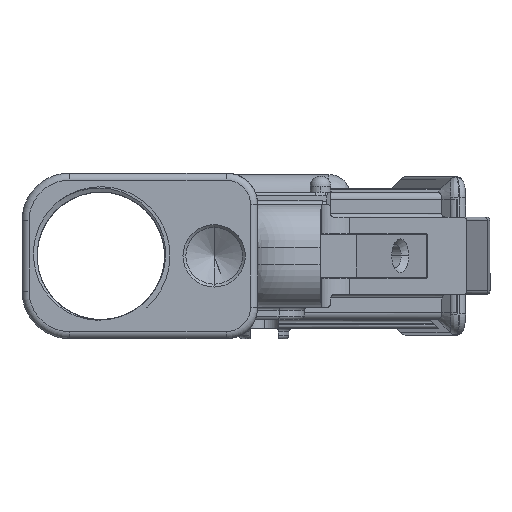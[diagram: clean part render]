
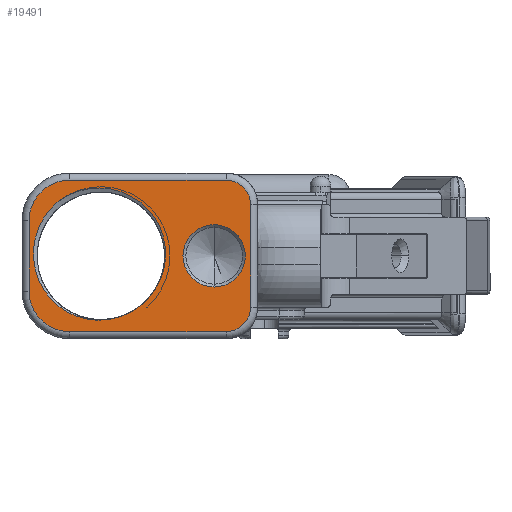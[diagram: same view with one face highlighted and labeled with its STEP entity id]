
A CAD part, left-side view. The second image highlights one B-rep face of the part: STEP entity #19491.
In plain terms, the highlighted planar face has unit normal (-1, 0, 0).
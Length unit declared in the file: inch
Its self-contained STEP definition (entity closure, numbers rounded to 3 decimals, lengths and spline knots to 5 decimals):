
#1840=DIRECTION('',(0.,0.,-1.));
#1841=VECTOR('',#1840,0.90625);
#1842=CARTESIAN_POINT('',(-7.565,-0.442,0.45313));
#1843=LINE('',#1842,#1841);
#1863=DIRECTION('',(0.,-1.,0.));
#1864=VECTOR('',#1863,1.38327);
#1865=CARTESIAN_POINT('',(-7.565,1.15661,0.66847));
#1866=LINE('',#1865,#1864);
#1882=DIRECTION('',(0.,0.,1.));
#1883=VECTOR('',#1882,0.62416);
#1884=CARTESIAN_POINT('',(-7.565,1.513,-0.31208));
#1885=LINE('',#1884,#1883);
#1890=CARTESIAN_POINT('',(-7.565,1.15661,-0.31208));
#1891=DIRECTION('',(-1.,0.,0.));
#1892=DIRECTION('',(0.,1.,0.));
#1893=AXIS2_PLACEMENT_3D('',#1890,#1891,#1892);
#1895=CARTESIAN_POINT('',(-7.565,1.15661,0.31208));
#1896=DIRECTION('',(-1.,0.,0.));
#1897=DIRECTION('',(0.,0.,1.));
#1898=AXIS2_PLACEMENT_3D('',#1895,#1896,#1897);
#1900=CARTESIAN_POINT('',(-7.565,-0.22666,0.45313));
#1901=DIRECTION('',(-1.,0.,0.));
#1902=DIRECTION('',(0.,-1.,0.));
#1903=AXIS2_PLACEMENT_3D('',#1900,#1901,#1902);
#1905=CARTESIAN_POINT('',(-7.565,-0.22666,-0.45313));
#1906=DIRECTION('',(-1.,0.,0.));
#1907=DIRECTION('',(0.,0.,-1.));
#1908=AXIS2_PLACEMENT_3D('',#1905,#1906,#1907);
#1910=CARTESIAN_POINT('',(-7.565,-0.1205,0.));
#1911=DIRECTION('',(1.,0.,0.));
#1912=DIRECTION('',(0.,0.,-1.));
#1913=AXIS2_PLACEMENT_3D('',#1910,#1911,#1912);
#1915=CARTESIAN_POINT('',(-7.565,-0.1205,0.));
#1916=DIRECTION('',(1.,0.,0.));
#1917=DIRECTION('',(0.,0.,1.));
#1918=AXIS2_PLACEMENT_3D('',#1915,#1916,#1917);
#1920=CARTESIAN_POINT('',(-7.565,0.8795,0.));
#1921=DIRECTION('',(1.,0.,0.));
#1922=DIRECTION('',(0.,-0.864,-0.503));
#1923=AXIS2_PLACEMENT_3D('',#1920,#1921,#1922);
#1925=DIRECTION('',(0.,1.,0.));
#1926=VECTOR('',#1925,1.38327);
#1927=CARTESIAN_POINT('',(-7.565,-0.22666,-0.66847));
#1928=LINE('',#1927,#1926);
#9167=CARTESIAN_POINT('',(-7.565,0.39331,-0.28289));
#9168=CARTESIAN_POINT('',(-7.565,0.37309,-0.2505));
#9169=CARTESIAN_POINT('',(-7.565,0.33995,-0.18304));
#9170=CARTESIAN_POINT('',(-7.565,0.31075,-0.07319));
#9171=CARTESIAN_POINT('',(-7.565,0.3044,0.04239));
#9172=CARTESIAN_POINT('',(-7.565,0.32039,0.15424));
#9173=CARTESIAN_POINT('',(-7.565,0.35858,0.26326));
#9174=CARTESIAN_POINT('',(-7.565,0.41751,0.36218));
#9175=CARTESIAN_POINT('',(-7.565,0.49489,0.44785));
#9176=CARTESIAN_POINT('',(-7.565,0.58856,0.51755));
#9177=CARTESIAN_POINT('',(-7.565,0.69295,0.56736));
#9178=CARTESIAN_POINT('',(-7.565,0.80785,0.5965));
#9179=CARTESIAN_POINT('',(-7.565,0.92518,0.60224));
#9180=CARTESIAN_POINT('',(-7.565,1.04407,0.58485));
#9181=CARTESIAN_POINT('',(-7.565,1.15676,0.54436));
#9182=CARTESIAN_POINT('',(-7.565,1.22454,0.50384));
#9183=CARTESIAN_POINT('',(-7.565,1.25678,0.47993));
#9207=CARTESIAN_POINT('',(-7.565,1.25678,0.47993));
#9208=CARTESIAN_POINT('',(-7.565,1.28795,0.45398));
#9209=CARTESIAN_POINT('',(-7.565,1.34373,0.39735));
#9210=CARTESIAN_POINT('',(-7.565,1.40926,
0.29779));
#9211=CARTESIAN_POINT('',(-7.565,1.45394,
0.18707));
#9212=CARTESIAN_POINT('',(-7.565,1.47587,
0.07176));
#9213=CARTESIAN_POINT('',(-7.565,1.4752,
-0.04651));
#9214=CARTESIAN_POINT('',(-7.565,1.4511,
-0.16151));
#9215=CARTESIAN_POINT('',(-7.565,1.4054,
-0.26861));
#9216=CARTESIAN_POINT('',(-7.565,1.339,
-0.36526));
#9217=CARTESIAN_POINT('',(-7.565,1.25645,
-0.44572));
#9218=CARTESIAN_POINT('',(-7.565,1.15841,
-0.50888));
#9219=CARTESIAN_POINT('',(-7.565,1.05132,
-0.55049));
#9220=CARTESIAN_POINT('',(-7.565,0.93705,
-0.5704));
#9221=CARTESIAN_POINT('',(-7.565,0.82106,
-0.56679));
#9222=CARTESIAN_POINT('',(-7.565,0.7483,
-0.5495));
#9223=CARTESIAN_POINT('',(-7.565,0.71257,
-0.53715));
#9616=CARTESIAN_POINT('',(-7.565,1.25678,0.47993));
#15622=CARTESIAN_POINT('',(-7.565,0.39331,-0.28289));
#15623=CARTESIAN_POINT('',(-7.565,0.71256,-0.53716));
#15624=VERTEX_POINT('',#15622);
#15625=VERTEX_POINT('',#15623);
#16979=VERTEX_POINT('',#9616);
#17004=CARTESIAN_POINT('',(-7.565,-0.22666,-0.66847));
#17005=CARTESIAN_POINT('',(-7.565,1.15661,-0.66847));
#17006=VERTEX_POINT('',#17004);
#17007=VERTEX_POINT('',#17005);
#17008=CARTESIAN_POINT('',(-7.565,-0.442,-0.45313));
#17009=VERTEX_POINT('',#17008);
#17010=CARTESIAN_POINT('',(-7.565,-0.442,0.45313));
#17011=VERTEX_POINT('',#17010);
#17012=CARTESIAN_POINT('',(-7.565,-0.22666,0.66847));
#17013=VERTEX_POINT('',#17012);
#17014=CARTESIAN_POINT('',(-7.565,1.15661,0.66847));
#17015=VERTEX_POINT('',#17014);
#17016=CARTESIAN_POINT('',(-7.565,1.513,0.31208));
#17017=VERTEX_POINT('',#17016);
#17018=CARTESIAN_POINT('',(-7.565,1.513,-0.31208));
#17019=VERTEX_POINT('',#17018);
#17020=CARTESIAN_POINT('',(-7.565,-0.1205,-0.275));
#17021=CARTESIAN_POINT('',(-7.565,-0.1205,0.275));
#17022=VERTEX_POINT('',#17020);
#17023=VERTEX_POINT('',#17021);
#19459=CARTESIAN_POINT('',(-7.565,0.,-0.45313));
#19460=DIRECTION('',(-1.,0.,0.));
#19461=DIRECTION('',(0.,0.,1.));
#19462=AXIS2_PLACEMENT_3D('',#19459,#19460,#19461);
#19463=PLANE('',#19462);
#19465=ORIENTED_EDGE('',*,*,#19464,.T.);
#19467=ORIENTED_EDGE('',*,*,#19466,.F.);
#19468=ORIENTED_EDGE('',*,*,#19450,.T.);
#19469=ORIENTED_EDGE('',*,*,#19439,.F.);
#19470=ORIENTED_EDGE('',*,*,#19424,.T.);
#19471=ORIENTED_EDGE('',*,*,#19409,.F.);
#19472=ORIENTED_EDGE('',*,*,#19394,.T.);
#19474=ORIENTED_EDGE('',*,*,#19473,.F.);
#19475=EDGE_LOOP('',(#19465,#19467,#19468,#19469,#19470,#19471,#19472,#19474));
#19476=FACE_OUTER_BOUND('',#19475,.F.);
#19478=ORIENTED_EDGE('',*,*,#19477,.F.);
#19480=ORIENTED_EDGE('',*,*,#19479,.F.);
#19481=EDGE_LOOP('',(#19478,#19480));
#19482=FACE_BOUND('',#19481,.F.);
#19484=ORIENTED_EDGE('',*,*,#19483,.T.);
#19486=ORIENTED_EDGE('',*,*,#19485,.F.);
#19488=ORIENTED_EDGE('',*,*,#19487,.T.);
#19489=EDGE_LOOP('',(#19484,#19486,#19488));
#19490=FACE_BOUND('',#19489,.F.);
#19491=ADVANCED_FACE('',(#19476,#19482,#19490),#19463,.T.);
#1894=CIRCLE('',#1893,0.35639);
#1899=CIRCLE('',#1898,0.35639);
#1904=CIRCLE('',#1903,0.21534);
#1909=CIRCLE('',#1908,0.21534);
#1914=CIRCLE('',#1913,0.275);
#1919=CIRCLE('',#1918,0.275);
#1924=CIRCLE('',#1923,0.5625);
#9184=B_SPLINE_CURVE_WITH_KNOTS('',3,(#9167,#9168,#9169,#9170,#9171,#9172,#9173,
#9174,#9175,#9176,#9177,#9178,#9179,#9180,#9181,#9182,#9183),.UNSPECIFIED.,.F.,
.F.,(4,1,1,1,1,1,1,1,1,1,1,1,1,1,4),(0.,0.07143,0.14286,
0.21429,0.28571,0.35714,0.42857,0.5,
0.57143,0.64286,0.71429,0.78571,
0.85714,0.92857,1.),.UNSPECIFIED.);
#9224=B_SPLINE_CURVE_WITH_KNOTS('',3,(#9207,#9208,#9209,#9210,#9211,#9212,#9213,
#9214,#9215,#9216,#9217,#9218,#9219,#9220,#9221,#9222,#9223),.UNSPECIFIED.,.F.,
.F.,(4,1,1,1,1,1,1,1,1,1,1,1,1,1,4),(0.,0.07143,0.14286,
0.21429,0.28571,0.35714,0.42857,0.5,
0.57143,0.64286,0.71429,0.78571,
0.85714,0.92857,1.),.UNSPECIFIED.);
#19394=EDGE_CURVE('',#17011,#17009,#1843,.T.);
#19409=EDGE_CURVE('',#17011,#17013,#1904,.T.);
#19424=EDGE_CURVE('',#17015,#17013,#1866,.T.);
#19439=EDGE_CURVE('',#17015,#17017,#1899,.T.);
#19450=EDGE_CURVE('',#17019,#17017,#1885,.T.);
#19464=EDGE_CURVE('',#17006,#17007,#1928,.T.);
#19466=EDGE_CURVE('',#17019,#17007,#1894,.T.);
#19473=EDGE_CURVE('',#17006,#17009,#1909,.T.);
#19477=EDGE_CURVE('',#17022,#17023,#1914,.T.);
#19479=EDGE_CURVE('',#17023,#17022,#1919,.T.);
#19483=EDGE_CURVE('',#16979,#15625,#9224,.T.);
#19485=EDGE_CURVE('',#15624,#15625,#1924,.T.);
#19487=EDGE_CURVE('',#15624,#16979,#9184,.T.);
